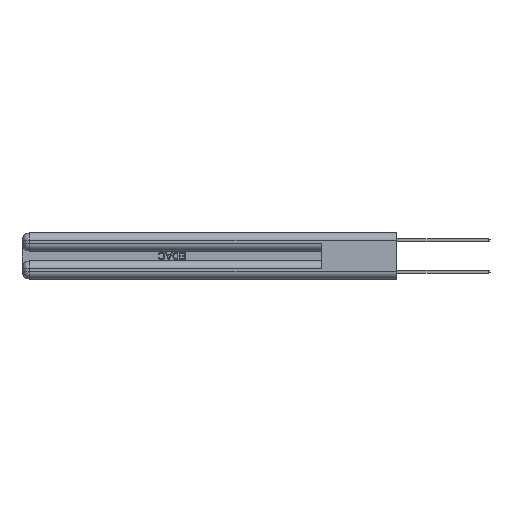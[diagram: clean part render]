
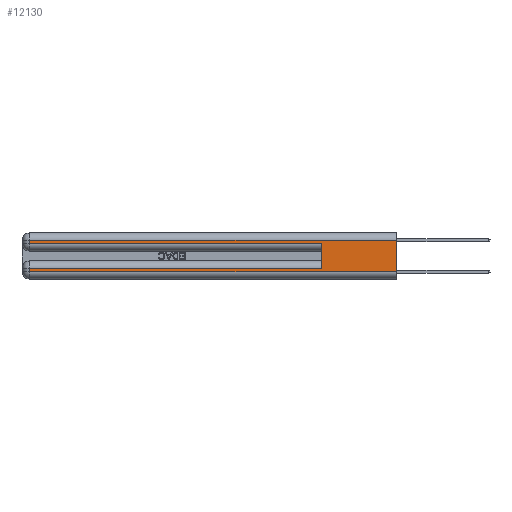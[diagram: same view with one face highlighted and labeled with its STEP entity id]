
A CAD part, left-side view. The second image highlights one B-rep face of the part: STEP entity #12130.
In plain terms, the highlighted planar face has unit normal (-1, 0, 0).
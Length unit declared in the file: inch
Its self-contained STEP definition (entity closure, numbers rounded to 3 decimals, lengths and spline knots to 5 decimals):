
#1024 = CARTESIAN_POINT ( 'NONE',  ( 0., 0., 0.06 ) ) ;
#1027 = DIRECTION ( 'NONE',  ( 0., 0., -1. ) ) ;
#1065 = EDGE_CURVE ( 'NONE', #16217, #26555, #3195, .T. ) ;
#1365 = CARTESIAN_POINT ( 'NONE',  ( 0., 2.94, 0.06 ) ) ;
#2159 = CARTESIAN_POINT ( 'NONE',  ( 0., 2.94, 0.37 ) ) ;
#2486 = DIRECTION ( 'NONE',  ( 0., 0., -1. ) ) ;
#2681 = EDGE_LOOP ( 'NONE', ( #26795, #31279, #3440, #14140, #16157, #32324, #17337, #7210 ) ) ;
#2968 = CARTESIAN_POINT ( 'NONE',  ( 0., 2.94, 0.31 ) ) ;
#3195 = LINE ( 'NONE', #10821, #6762 ) ;
#3440 = ORIENTED_EDGE ( 'NONE', *, *, #4298, .T. ) ;
#4298 = EDGE_CURVE ( 'NONE', #18746, #28371, #27223, .T. ) ;
#4558 = VERTEX_POINT ( 'NONE', #23583 ) ;
#5443 = LINE ( 'NONE', #13753, #29150 ) ;
#5949 = VECTOR ( 'NONE', #11224, 39.37008 ) ;
#6762 = VECTOR ( 'NONE', #21825, 39.37008 ) ;
#7210 = ORIENTED_EDGE ( 'NONE', *, *, #11585, .T. ) ;
#8092 = CARTESIAN_POINT ( 'NONE',  ( 0., 2.94, 0.37 ) ) ;
#8218 = DIRECTION ( 'NONE',  ( 0., -1., 0. ) ) ;
#8838 = EDGE_CURVE ( 'NONE', #28371, #29991, #32955, .T. ) ;
#9068 = CARTESIAN_POINT ( 'NONE',  ( 0., 0.6, 0.285 ) ) ;
#10133 = CARTESIAN_POINT ( 'NONE',  ( 0., 0., 0.31 ) ) ;
#10786 = VECTOR ( 'NONE', #21306, 39.37008 ) ;
#10821 = CARTESIAN_POINT ( 'NONE',  ( 0., 0., 0.37 ) ) ;
#11224 = DIRECTION ( 'NONE',  ( 0., 0., 1. ) ) ;
#11585 = EDGE_CURVE ( 'NONE', #21919, #26555, #17472, .T. ) ;
#11934 = CARTESIAN_POINT ( 'NONE',  ( 0., 0.6, 0.145 ) ) ;
#12130 = ADVANCED_FACE ( 'NONE', ( #28469 ), #14767, .F. ) ;
#12417 = CARTESIAN_POINT ( 'NONE',  ( 0., 0., 0.37 ) ) ;
#13753 = CARTESIAN_POINT ( 'NONE',  ( 0., 0., 0.31 ) ) ;
#14140 = ORIENTED_EDGE ( 'NONE', *, *, #8838, .T. ) ;
#14767 = PLANE ( 'NONE',  #33654 ) ;
#15973 = CARTESIAN_POINT ( 'NONE',  ( 0., 0., 0.085 ) ) ;
#16157 = ORIENTED_EDGE ( 'NONE', *, *, #31775, .F. ) ;
#16217 = VERTEX_POINT ( 'NONE', #10133 ) ;
#16259 = LINE ( 'NONE', #2159, #10786 ) ;
#17211 = VECTOR ( 'NONE', #2486, 39.37008 ) ;
#17337 = ORIENTED_EDGE ( 'NONE', *, *, #22386, .T. ) ;
#17472 = LINE ( 'NONE', #1024, #26130 ) ;
#18020 = DIRECTION ( 'NONE',  ( 1., 0., 0. ) ) ;
#18690 = DIRECTION ( 'NONE',  ( 0., 1., 0. ) ) ;
#18746 = VERTEX_POINT ( 'NONE', #2968 ) ;
#20742 = EDGE_CURVE ( 'NONE', #16217, #18746, #5443, .T. ) ;
#21306 = DIRECTION ( 'NONE',  ( 0., 0., -1. ) ) ;
#21825 = DIRECTION ( 'NONE',  ( 0., 0., -1. ) ) ;
#21919 = VERTEX_POINT ( 'NONE', #1365 ) ;
#22386 = EDGE_CURVE ( 'NONE', #4558, #21919, #16259, .T. ) ;
#23052 = DIRECTION ( 'NONE',  ( 0., -1., 0. ) ) ;
#23583 = CARTESIAN_POINT ( 'NONE',  ( 0., 2.94, 0.085 ) ) ;
#24754 = DIRECTION ( 'NONE',  ( 0., 1., 0. ) ) ;
#25639 = LINE ( 'NONE', #11934, #5949 ) ;
#26130 = VECTOR ( 'NONE', #23052, 39.37008 ) ;
#26555 = VERTEX_POINT ( 'NONE', #31891 ) ;
#26795 = ORIENTED_EDGE ( 'NONE', *, *, #1065, .F. ) ;
#27223 = LINE ( 'NONE', #8092, #17211 ) ;
#28321 = VECTOR ( 'NONE', #18690, 39.37008 ) ;
#28371 = VERTEX_POINT ( 'NONE', #35080 ) ;
#28469 = FACE_OUTER_BOUND ( 'NONE', #2681, .T. ) ;
#29150 = VECTOR ( 'NONE', #24754, 39.37008 ) ;
#29790 = EDGE_CURVE ( 'NONE', #32731, #4558, #30042, .T. ) ;
#29881 = CARTESIAN_POINT ( 'NONE',  ( 0., 0., 0.285 ) ) ;
#29991 = VERTEX_POINT ( 'NONE', #9068 ) ;
#30042 = LINE ( 'NONE', #15973, #28321 ) ;
#31279 = ORIENTED_EDGE ( 'NONE', *, *, #20742, .T. ) ;
#31775 = EDGE_CURVE ( 'NONE', #32731, #29991, #25639, .T. ) ;
#31891 = CARTESIAN_POINT ( 'NONE',  ( 0., 0., 0.06 ) ) ;
#32324 = ORIENTED_EDGE ( 'NONE', *, *, #29790, .T. ) ;
#32731 = VERTEX_POINT ( 'NONE', #34730 ) ;
#32955 = LINE ( 'NONE', #29881, #33573 ) ;
#33573 = VECTOR ( 'NONE', #8218, 39.37008 ) ;
#33654 = AXIS2_PLACEMENT_3D ( 'NONE', #12417, #18020, #1027 ) ;
#34730 = CARTESIAN_POINT ( 'NONE',  ( 0., 0.6, 0.085 ) ) ;
#35080 = CARTESIAN_POINT ( 'NONE',  ( 0., 2.94, 0.285 ) ) ;
